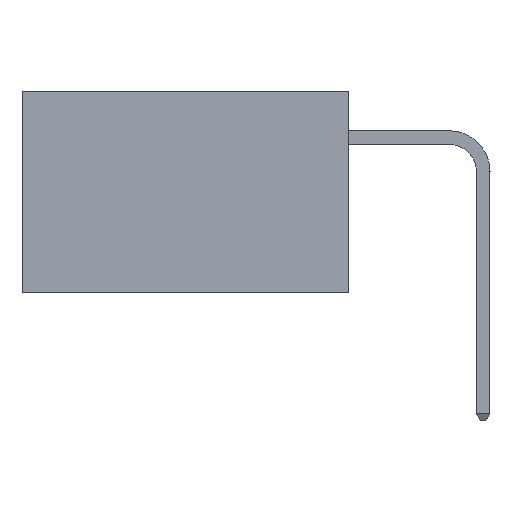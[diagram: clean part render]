
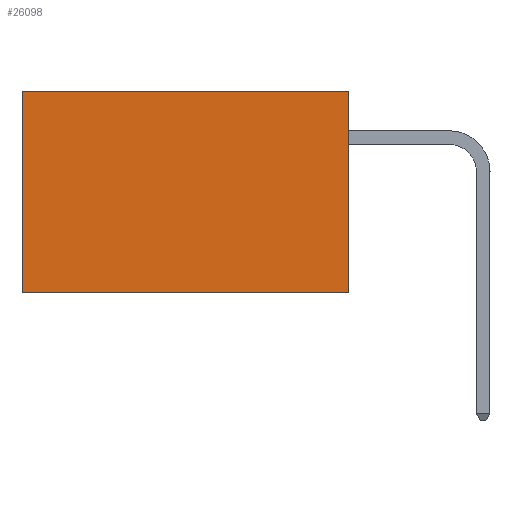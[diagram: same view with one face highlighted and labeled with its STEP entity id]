
A CAD part, left-side view. The second image highlights one B-rep face of the part: STEP entity #26098.
In plain terms, the highlighted planar face has unit normal (-1, 0, 0).
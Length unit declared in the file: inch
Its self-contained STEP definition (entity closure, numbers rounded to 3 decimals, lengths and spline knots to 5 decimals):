
#1799 = VERTEX_POINT ( 'NONE', #8777 ) ;
#2640 = VECTOR ( 'NONE', #16130, 39.37008 ) ;
#2935 = CARTESIAN_POINT ( 'NONE',  ( 0.2875, 0.6, 0. ) ) ;
#3790 = VERTEX_POINT ( 'NONE', #2935 ) ;
#3929 = CARTESIAN_POINT ( 'NONE',  ( 0.2875, 0., -0.37 ) ) ;
#5973 = CARTESIAN_POINT ( 'NONE',  ( 0.2875, 0., -0.37 ) ) ;
#6544 = DIRECTION ( 'NONE',  ( 0., 0., -1. ) ) ;
#8540 = EDGE_LOOP ( 'NONE', ( #31508, #10037, #24787, #28318 ) ) ;
#8777 = CARTESIAN_POINT ( 'NONE',  ( 0.2875, 0., 0. ) ) ;
#8902 = LINE ( 'NONE', #23930, #22844 ) ;
#9258 = CARTESIAN_POINT ( 'NONE',  ( 0.2875, 0., 0. ) ) ;
#10037 = ORIENTED_EDGE ( 'NONE', *, *, #21828, .F. ) ;
#11190 = VERTEX_POINT ( 'NONE', #33084 ) ;
#12867 = DIRECTION ( 'NONE',  ( 0., 1., 0. ) ) ;
#13089 = VECTOR ( 'NONE', #25677, 39.37008 ) ;
#16130 = DIRECTION ( 'NONE',  ( 0., 0., -1. ) ) ;
#18092 = AXIS2_PLACEMENT_3D ( 'NONE', #9258, #23259, #6544 ) ;
#18646 = VERTEX_POINT ( 'NONE', #3929 ) ;
#21828 = EDGE_CURVE ( 'NONE', #18646, #11190, #27001, .T. ) ;
#22843 = CARTESIAN_POINT ( 'NONE',  ( 0.2875, 0.6, 0. ) ) ;
#22844 = VECTOR ( 'NONE', #12867, 39.37008 ) ;
#23259 = DIRECTION ( 'NONE',  ( 1., 0., 0. ) ) ;
#23930 = CARTESIAN_POINT ( 'NONE',  ( 0.2875, 0., 0. ) ) ;
#24351 = FACE_OUTER_BOUND ( 'NONE', #8540, .T. ) ;
#24683 = EDGE_CURVE ( 'NONE', #3790, #11190, #27042, .T. ) ;
#24787 = ORIENTED_EDGE ( 'NONE', *, *, #33701, .F. ) ;
#24933 = LINE ( 'NONE', #27264, #2640 ) ;
#25514 = DIRECTION ( 'NONE',  ( 0., 1., 0. ) ) ;
#25677 = DIRECTION ( 'NONE',  ( 0., 0., -1. ) ) ;
#26098 = ADVANCED_FACE ( 'NONE', ( #24351 ), #34281, .F. ) ;
#27001 = LINE ( 'NONE', #5973, #33487 ) ;
#27042 = LINE ( 'NONE', #22843, #13089 ) ;
#27264 = CARTESIAN_POINT ( 'NONE',  ( 0.2875, 0., 0. ) ) ;
#28318 = ORIENTED_EDGE ( 'NONE', *, *, #32249, .T. ) ;
#31508 = ORIENTED_EDGE ( 'NONE', *, *, #24683, .T. ) ;
#32249 = EDGE_CURVE ( 'NONE', #1799, #3790, #8902, .T. ) ;
#33084 = CARTESIAN_POINT ( 'NONE',  ( 0.2875, 0.6, -0.37 ) ) ;
#33487 = VECTOR ( 'NONE', #25514, 39.37008 ) ;
#33701 = EDGE_CURVE ( 'NONE', #1799, #18646, #24933, .T. ) ;
#34281 = PLANE ( 'NONE',  #18092 ) ;
